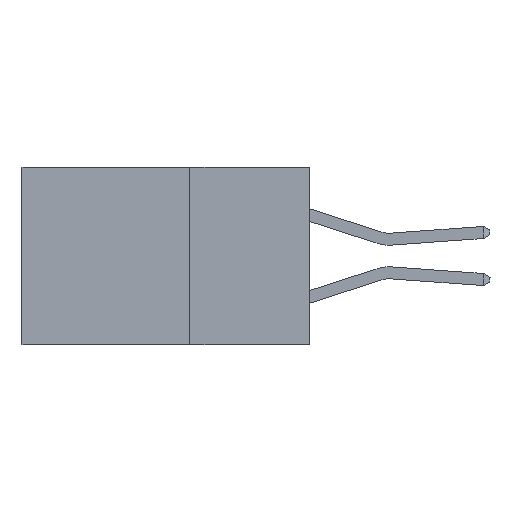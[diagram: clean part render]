
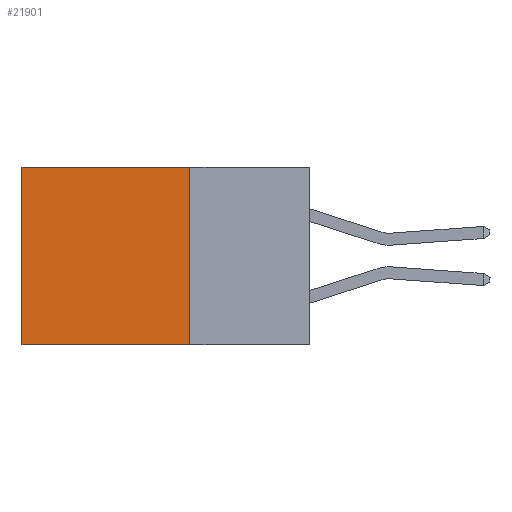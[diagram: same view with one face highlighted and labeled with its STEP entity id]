
A CAD part, left-side view. The second image highlights one B-rep face of the part: STEP entity #21901.
In plain terms, the highlighted planar face has unit normal (-1, 0, 0).
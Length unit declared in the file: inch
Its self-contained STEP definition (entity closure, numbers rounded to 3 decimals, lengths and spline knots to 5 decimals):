
#575 = CARTESIAN_POINT ( 'NONE',  ( 0.298, 0.25, 0. ) ) ;
#3947 = DIRECTION ( 'NONE',  ( 0., 1., 0. ) ) ;
#4038 = CARTESIAN_POINT ( 'NONE',  ( 0.298, 0.25, -0.37 ) ) ;
#4684 = VECTOR ( 'NONE', #3947, 39.37008 ) ;
#5797 = CARTESIAN_POINT ( 'NONE',  ( 0.298, 0.25, -0.37 ) ) ;
#5925 = VERTEX_POINT ( 'NONE', #4038 ) ;
#6049 = LINE ( 'NONE', #5797, #4684 ) ;
#6375 = VERTEX_POINT ( 'NONE', #8596 ) ;
#7698 = CARTESIAN_POINT ( 'NONE',  ( 0.298, 0.6, -0.37 ) ) ;
#8229 = AXIS2_PLACEMENT_3D ( 'NONE', #8625, #14233, #20948 ) ;
#8596 = CARTESIAN_POINT ( 'NONE',  ( 0.298, 0.25, 0. ) ) ;
#8625 = CARTESIAN_POINT ( 'NONE',  ( 0.298, 0.25, 0. ) ) ;
#9670 = VECTOR ( 'NONE', #17806, 39.37008 ) ;
#12971 = DIRECTION ( 'NONE',  ( 0., 0., -1. ) ) ;
#13782 = EDGE_CURVE ( 'NONE', #6375, #19185, #22085, .T. ) ;
#14233 = DIRECTION ( 'NONE',  ( 1., 0., 0. ) ) ;
#14381 = LINE ( 'NONE', #575, #21761 ) ;
#15064 = VERTEX_POINT ( 'NONE', #7698 ) ;
#15711 = DIRECTION ( 'NONE',  ( 0., 0., -1. ) ) ;
#16117 = CARTESIAN_POINT ( 'NONE',  ( 0.298, 0.25, 0. ) ) ;
#16830 = ORIENTED_EDGE ( 'NONE', *, *, #21407, .F. ) ;
#17806 = DIRECTION ( 'NONE',  ( 0., 1., 0. ) ) ;
#17842 = EDGE_LOOP ( 'NONE', ( #20346, #20398, #16830, #18822 ) ) ;
#18822 = ORIENTED_EDGE ( 'NONE', *, *, #13782, .T. ) ;
#19185 = VERTEX_POINT ( 'NONE', #21219 ) ;
#19891 = VECTOR ( 'NONE', #15711, 39.37008 ) ;
#20007 = EDGE_CURVE ( 'NONE', #19185, #15064, #22367, .T. ) ;
#20346 = ORIENTED_EDGE ( 'NONE', *, *, #20007, .T. ) ;
#20398 = ORIENTED_EDGE ( 'NONE', *, *, #21371, .F. ) ;
#20824 = CARTESIAN_POINT ( 'NONE',  ( 0.298, 0.6, 0. ) ) ;
#20948 = DIRECTION ( 'NONE',  ( 0., 0., -1. ) ) ;
#21219 = CARTESIAN_POINT ( 'NONE',  ( 0.298, 0.6, 0. ) ) ;
#21371 = EDGE_CURVE ( 'NONE', #5925, #15064, #6049, .T. ) ;
#21407 = EDGE_CURVE ( 'NONE', #6375, #5925, #14381, .T. ) ;
#21761 = VECTOR ( 'NONE', #12971, 39.37008 ) ;
#21901 = ADVANCED_FACE ( 'NONE', ( #22265 ), #22739, .F. ) ;
#22085 = LINE ( 'NONE', #16117, #9670 ) ;
#22265 = FACE_OUTER_BOUND ( 'NONE', #17842, .T. ) ;
#22367 = LINE ( 'NONE', #20824, #19891 ) ;
#22739 = PLANE ( 'NONE',  #8229 ) ;
